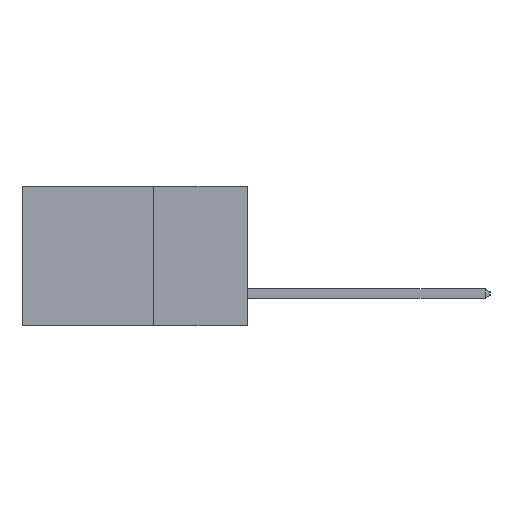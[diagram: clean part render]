
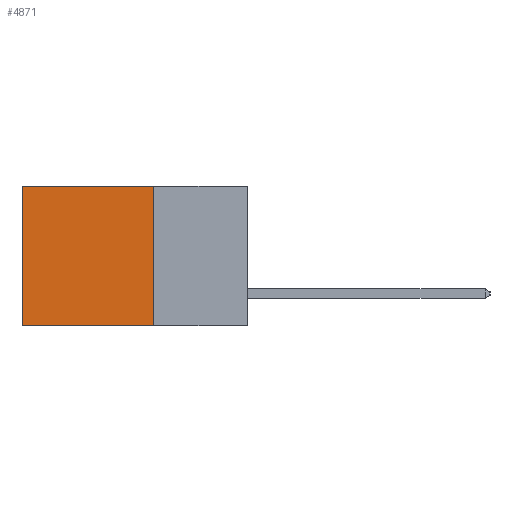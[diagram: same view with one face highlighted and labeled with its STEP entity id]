
A CAD part, left-side view. The second image highlights one B-rep face of the part: STEP entity #4871.
In plain terms, the highlighted planar face has unit normal (-1, 0, 0).
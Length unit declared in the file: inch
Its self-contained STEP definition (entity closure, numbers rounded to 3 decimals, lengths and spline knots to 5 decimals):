
#696 = DIRECTION ( 'NONE',  ( 0., 0., -1. ) ) ;
#723 = CARTESIAN_POINT ( 'NONE',  ( 0.2615, 0.6, -0.37 ) ) ;
#847 = CARTESIAN_POINT ( 'NONE',  ( 0.2615, 0.25, -0.37 ) ) ;
#987 = CARTESIAN_POINT ( 'NONE',  ( 0.2615, 0.25, 0. ) ) ;
#1275 = DIRECTION ( 'NONE',  ( 0., 0., -1. ) ) ;
#1314 = ORIENTED_EDGE ( 'NONE', *, *, #4526, .T. ) ;
#1824 = EDGE_CURVE ( 'NONE', #2120, #7727, #12073, .T. ) ;
#2025 = LINE ( 'NONE', #5125, #11950 ) ;
#2120 = VERTEX_POINT ( 'NONE', #10540 ) ;
#2333 = VERTEX_POINT ( 'NONE', #987 ) ;
#3268 = CARTESIAN_POINT ( 'NONE',  ( 0.2615, 0.6, -0.37 ) ) ;
#3565 = ORIENTED_EDGE ( 'NONE', *, *, #1824, .T. ) ;
#4271 = VECTOR ( 'NONE', #1275, 39.37008 ) ;
#4447 = AXIS2_PLACEMENT_3D ( 'NONE', #12594, #6841, #696 ) ;
#4526 = EDGE_CURVE ( 'NONE', #2333, #2120, #8003, .T. ) ;
#4871 = ADVANCED_FACE ( 'NONE', ( #9529 ), #5822, .F. ) ;
#4985 = VERTEX_POINT ( 'NONE', #8670 ) ;
#5125 = CARTESIAN_POINT ( 'NONE',  ( 0.2615, 0.25, -0.37 ) ) ;
#5257 = CARTESIAN_POINT ( 'NONE',  ( 0.2615, 0.25, 0. ) ) ;
#5822 = PLANE ( 'NONE',  #4447 ) ;
#5958 = VECTOR ( 'NONE', #12109, 39.37008 ) ;
#6053 = LINE ( 'NONE', #847, #8402 ) ;
#6841 = DIRECTION ( 'NONE',  ( 1., 0., 0. ) ) ;
#7727 = VERTEX_POINT ( 'NONE', #723 ) ;
#8003 = LINE ( 'NONE', #5257, #5958 ) ;
#8267 = ORIENTED_EDGE ( 'NONE', *, *, #8867, .F. ) ;
#8402 = VECTOR ( 'NONE', #8996, 39.37008 ) ;
#8670 = CARTESIAN_POINT ( 'NONE',  ( 0.2615, 0.25, -0.37 ) ) ;
#8867 = EDGE_CURVE ( 'NONE', #2333, #4985, #6053, .T. ) ;
#8996 = DIRECTION ( 'NONE',  ( 0., 0., -1. ) ) ;
#9529 = FACE_OUTER_BOUND ( 'NONE', #12534, .T. ) ;
#10540 = CARTESIAN_POINT ( 'NONE',  ( 0.2615, 0.6, 0. ) ) ;
#11029 = DIRECTION ( 'NONE',  ( 0., 1., 0. ) ) ;
#11498 = ORIENTED_EDGE ( 'NONE', *, *, #12617, .F. ) ;
#11950 = VECTOR ( 'NONE', #11029, 39.37008 ) ;
#12073 = LINE ( 'NONE', #3268, #4271 ) ;
#12109 = DIRECTION ( 'NONE',  ( 0., 1., 0. ) ) ;
#12534 = EDGE_LOOP ( 'NONE', ( #3565, #11498, #8267, #1314 ) ) ;
#12594 = CARTESIAN_POINT ( 'NONE',  ( 0.2615, 0.25, -0.37 ) ) ;
#12617 = EDGE_CURVE ( 'NONE', #4985, #7727, #2025, .T. ) ;
